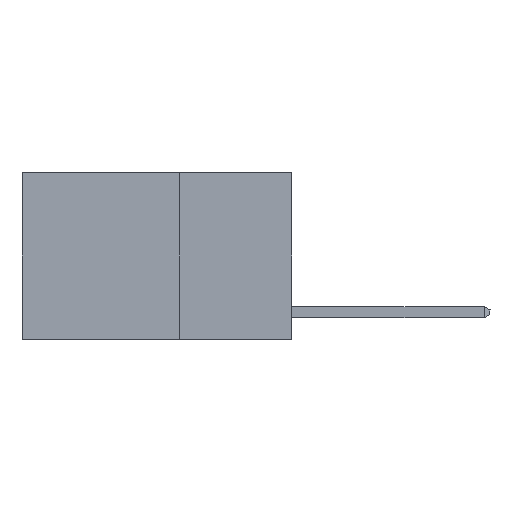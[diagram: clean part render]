
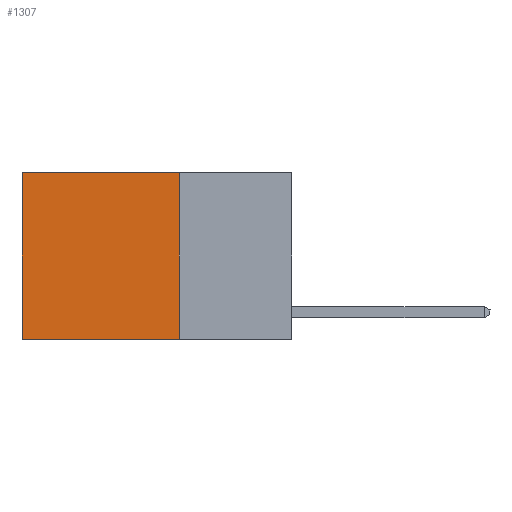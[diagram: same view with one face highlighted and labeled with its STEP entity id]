
A CAD part, left-side view. The second image highlights one B-rep face of the part: STEP entity #1307.
In plain terms, the highlighted planar face has unit normal (-1, 0, 0).
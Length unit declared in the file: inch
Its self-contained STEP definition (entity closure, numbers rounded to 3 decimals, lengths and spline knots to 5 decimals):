
#414 = ORIENTED_EDGE ( 'NONE', *, *, #12590, .T. ) ;
#765 = ORIENTED_EDGE ( 'NONE', *, *, #6161, .F. ) ;
#1307 = ADVANCED_FACE ( 'NONE', ( #26263 ), #6437, .F. ) ;
#1613 = VERTEX_POINT ( 'NONE', #18742 ) ;
#1888 = CARTESIAN_POINT ( 'NONE',  ( 0.2625, 0.6, -0.37 ) ) ;
#1939 = VECTOR ( 'NONE', #6190, 39.37008 ) ;
#2491 = DIRECTION ( 'NONE',  ( 0., 1., 0. ) ) ;
#2546 = CARTESIAN_POINT ( 'NONE',  ( 0.2625, 0.6, 0. ) ) ;
#2573 = CARTESIAN_POINT ( 'NONE',  ( 0.2625, 0.25, -0.37 ) ) ;
#3511 = EDGE_LOOP ( 'NONE', ( #4443, #765, #7129, #414 ) ) ;
#3958 = LINE ( 'NONE', #2573, #18626 ) ;
#4225 = DIRECTION ( 'NONE',  ( 0., 0., -1. ) ) ;
#4443 = ORIENTED_EDGE ( 'NONE', *, *, #16111, .T. ) ;
#5170 = CARTESIAN_POINT ( 'NONE',  ( 0.2625, 0.25, 0. ) ) ;
#6043 = LINE ( 'NONE', #5170, #26865 ) ;
#6161 = EDGE_CURVE ( 'NONE', #21165, #6628, #3958, .T. ) ;
#6190 = DIRECTION ( 'NONE',  ( 0., 0., -1. ) ) ;
#6403 = DIRECTION ( 'NONE',  ( 1., 0., 0. ) ) ;
#6437 = PLANE ( 'NONE',  #16558 ) ;
#6628 = VERTEX_POINT ( 'NONE', #1888 ) ;
#7129 = ORIENTED_EDGE ( 'NONE', *, *, #16927, .F. ) ;
#8199 = LINE ( 'NONE', #14540, #1939 ) ;
#9219 = VERTEX_POINT ( 'NONE', #2546 ) ;
#10356 = VECTOR ( 'NONE', #2491, 39.37008 ) ;
#12590 = EDGE_CURVE ( 'NONE', #1613, #9219, #26949, .T. ) ;
#14540 = CARTESIAN_POINT ( 'NONE',  ( 0.2625, 0.6, 0. ) ) ;
#16111 = EDGE_CURVE ( 'NONE', #9219, #6628, #8199, .T. ) ;
#16461 = CARTESIAN_POINT ( 'NONE',  ( 0.2625, 0.25, 0. ) ) ;
#16558 = AXIS2_PLACEMENT_3D ( 'NONE', #16461, #6403, #4225 ) ;
#16927 = EDGE_CURVE ( 'NONE', #1613, #21165, #6043, .T. ) ;
#18626 = VECTOR ( 'NONE', #19292, 39.37008 ) ;
#18742 = CARTESIAN_POINT ( 'NONE',  ( 0.2625, 0.25, 0. ) ) ;
#19292 = DIRECTION ( 'NONE',  ( 0., 1., 0. ) ) ;
#21165 = VERTEX_POINT ( 'NONE', #25190 ) ;
#23279 = CARTESIAN_POINT ( 'NONE',  ( 0.2625, 0.25, 0. ) ) ;
#25190 = CARTESIAN_POINT ( 'NONE',  ( 0.2625, 0.25, -0.37 ) ) ;
#25999 = DIRECTION ( 'NONE',  ( 0., 0., -1. ) ) ;
#26263 = FACE_OUTER_BOUND ( 'NONE', #3511, .T. ) ;
#26865 = VECTOR ( 'NONE', #25999, 39.37008 ) ;
#26949 = LINE ( 'NONE', #23279, #10356 ) ;
